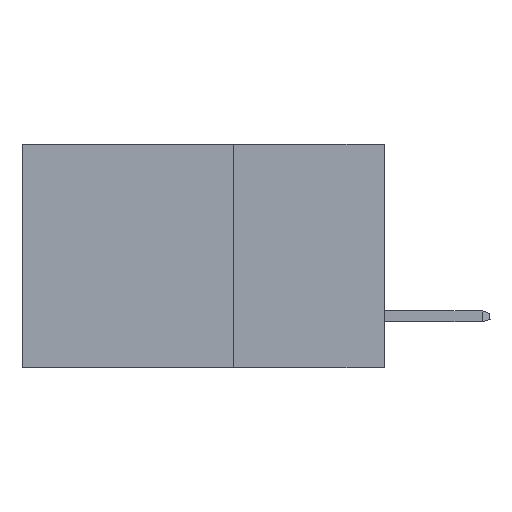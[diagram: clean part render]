
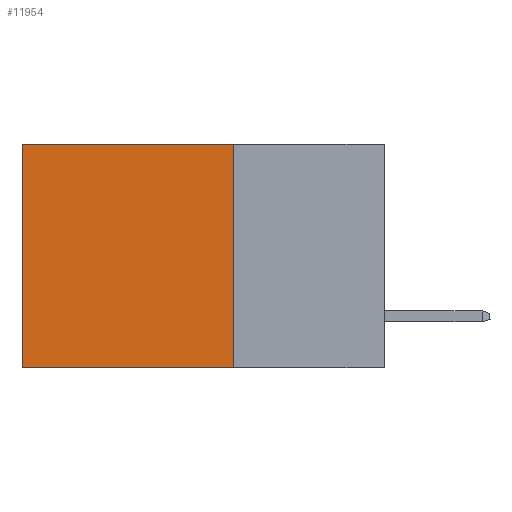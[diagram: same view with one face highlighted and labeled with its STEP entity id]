
A CAD part, left-side view. The second image highlights one B-rep face of the part: STEP entity #11954.
In plain terms, the highlighted planar face has unit normal (-1, 0, 0).
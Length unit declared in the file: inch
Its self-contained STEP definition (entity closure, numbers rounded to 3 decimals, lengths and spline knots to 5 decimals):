
#396 = ORIENTED_EDGE ( 'NONE', *, *, #15439, .F. ) ;
#2262 = VECTOR ( 'NONE', #11426, 39.37008 ) ;
#2671 = VERTEX_POINT ( 'NONE', #3121 ) ;
#3121 = CARTESIAN_POINT ( 'NONE',  ( 0.298, 0.25, -0.37 ) ) ;
#3421 = CARTESIAN_POINT ( 'NONE',  ( 0.298, 0.25, 0. ) ) ;
#4212 = CARTESIAN_POINT ( 'NONE',  ( 0.298, 0.6, 0. ) ) ;
#5535 = VECTOR ( 'NONE', #8519, 39.37008 ) ;
#6136 = LINE ( 'NONE', #9441, #5535 ) ;
#8400 = DIRECTION ( 'NONE',  ( 0., 0., -1. ) ) ;
#8519 = DIRECTION ( 'NONE',  ( 0., 0., -1. ) ) ;
#8723 = CARTESIAN_POINT ( 'NONE',  ( 0.298, 0.25, 0. ) ) ;
#9297 = EDGE_CURVE ( 'NONE', #11077, #19175, #6136, .T. ) ;
#9441 = CARTESIAN_POINT ( 'NONE',  ( 0.298, 0.6, 0. ) ) ;
#10743 = EDGE_LOOP ( 'NONE', ( #16735, #22915, #396, #12410 ) ) ;
#10749 = DIRECTION ( 'NONE',  ( 0., 0., -1. ) ) ;
#10797 = VECTOR ( 'NONE', #8400, 39.37008 ) ;
#11077 = VERTEX_POINT ( 'NONE', #4212 ) ;
#11426 = DIRECTION ( 'NONE',  ( 0., 1., 0. ) ) ;
#11922 = LINE ( 'NONE', #3421, #2262 ) ;
#11954 = ADVANCED_FACE ( 'NONE', ( #24395 ), #16406, .F. ) ;
#12060 = CARTESIAN_POINT ( 'NONE',  ( 0.298, 0.25, -0.37 ) ) ;
#12218 = EDGE_CURVE ( 'NONE', #12396, #11077, #11922, .T. ) ;
#12396 = VERTEX_POINT ( 'NONE', #21962 ) ;
#12410 = ORIENTED_EDGE ( 'NONE', *, *, #12218, .T. ) ;
#13920 = CARTESIAN_POINT ( 'NONE',  ( 0.298, 0.25, 0. ) ) ;
#15439 = EDGE_CURVE ( 'NONE', #12396, #2671, #15772, .T. ) ;
#15772 = LINE ( 'NONE', #13920, #10797 ) ;
#16406 = PLANE ( 'NONE',  #17441 ) ;
#16735 = ORIENTED_EDGE ( 'NONE', *, *, #9297, .T. ) ;
#17441 = AXIS2_PLACEMENT_3D ( 'NONE', #8723, #22670, #10749 ) ;
#18454 = LINE ( 'NONE', #12060, #20649 ) ;
#19175 = VERTEX_POINT ( 'NONE', #23497 ) ;
#20649 = VECTOR ( 'NONE', #22084, 39.37008 ) ;
#21962 = CARTESIAN_POINT ( 'NONE',  ( 0.298, 0.25, 0. ) ) ;
#22084 = DIRECTION ( 'NONE',  ( 0., 1., 0. ) ) ;
#22670 = DIRECTION ( 'NONE',  ( 1., 0., 0. ) ) ;
#22915 = ORIENTED_EDGE ( 'NONE', *, *, #23103, .F. ) ;
#23103 = EDGE_CURVE ( 'NONE', #2671, #19175, #18454, .T. ) ;
#23497 = CARTESIAN_POINT ( 'NONE',  ( 0.298, 0.6, -0.37 ) ) ;
#24395 = FACE_OUTER_BOUND ( 'NONE', #10743, .T. ) ;
